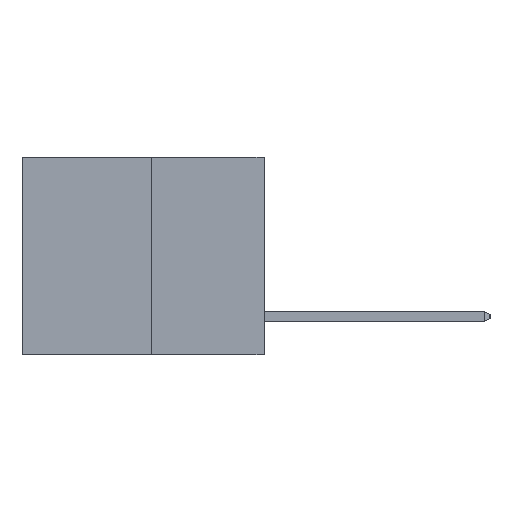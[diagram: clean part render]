
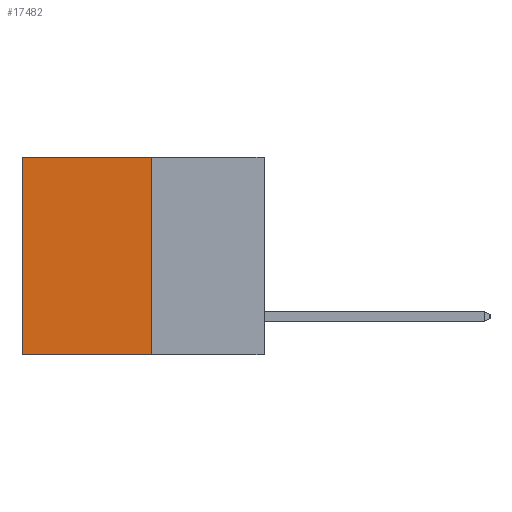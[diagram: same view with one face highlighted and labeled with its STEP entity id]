
A CAD part, left-side view. The second image highlights one B-rep face of the part: STEP entity #17482.
In plain terms, the highlighted planar face has unit normal (-1, 0, 0).
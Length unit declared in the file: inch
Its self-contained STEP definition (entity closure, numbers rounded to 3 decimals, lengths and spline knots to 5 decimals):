
#106 = ORIENTED_EDGE ( 'NONE', *, *, #21709, .F. ) ;
#440 = LINE ( 'NONE', #17711, #22484 ) ;
#1075 = CARTESIAN_POINT ( 'NONE',  ( 0.3165, 0.28, -0.49 ) ) ;
#2666 = DIRECTION ( 'NONE',  ( 0., 0., -1. ) ) ;
#2783 = EDGE_CURVE ( 'NONE', #6957, #25346, #440, .T. ) ;
#4240 = AXIS2_PLACEMENT_3D ( 'NONE', #26062, #8800, #26153 ) ;
#4554 = ORIENTED_EDGE ( 'NONE', *, *, #2783, .T. ) ;
#4633 = CARTESIAN_POINT ( 'NONE',  ( 0.3165, 0.28, 0. ) ) ;
#5804 = CARTESIAN_POINT ( 'NONE',  ( 0.3165, 0.28, 0. ) ) ;
#6434 = LINE ( 'NONE', #1075, #15392 ) ;
#6830 = EDGE_CURVE ( 'NONE', #8191, #25847, #21156, .T. ) ;
#6957 = VERTEX_POINT ( 'NONE', #19148 ) ;
#7073 = PLANE ( 'NONE',  #4240 ) ;
#8191 = VERTEX_POINT ( 'NONE', #5804 ) ;
#8423 = LINE ( 'NONE', #4633, #14415 ) ;
#8800 = DIRECTION ( 'NONE',  ( 1., 0., 0. ) ) ;
#9578 = CARTESIAN_POINT ( 'NONE',  ( 0.3165, 0.6, -0.49 ) ) ;
#11129 = ORIENTED_EDGE ( 'NONE', *, *, #6830, .F. ) ;
#13518 = EDGE_LOOP ( 'NONE', ( #4554, #106, #11129, #23353 ) ) ;
#14415 = VECTOR ( 'NONE', #17722, 39.37008 ) ;
#15269 = CARTESIAN_POINT ( 'NONE',  ( 0.3165, 0.28, -0.49 ) ) ;
#15392 = VECTOR ( 'NONE', #15847, 39.37008 ) ;
#15847 = DIRECTION ( 'NONE',  ( 0., 1., 0. ) ) ;
#15985 = CARTESIAN_POINT ( 'NONE',  ( 0.3165, 0.28, -0.49 ) ) ;
#17482 = ADVANCED_FACE ( 'NONE', ( #21801 ), #7073, .F. ) ;
#17711 = CARTESIAN_POINT ( 'NONE',  ( 0.3165, 0.6, -0.49 ) ) ;
#17722 = DIRECTION ( 'NONE',  ( 0., 1., 0. ) ) ;
#18143 = VECTOR ( 'NONE', #22916, 39.37008 ) ;
#19148 = CARTESIAN_POINT ( 'NONE',  ( 0.3165, 0.6, 0. ) ) ;
#21156 = LINE ( 'NONE', #15985, #18143 ) ;
#21499 = EDGE_CURVE ( 'NONE', #8191, #6957, #8423, .T. ) ;
#21709 = EDGE_CURVE ( 'NONE', #25847, #25346, #6434, .T. ) ;
#21801 = FACE_OUTER_BOUND ( 'NONE', #13518, .T. ) ;
#22484 = VECTOR ( 'NONE', #2666, 39.37008 ) ;
#22916 = DIRECTION ( 'NONE',  ( 0., 0., -1. ) ) ;
#23353 = ORIENTED_EDGE ( 'NONE', *, *, #21499, .T. ) ;
#25346 = VERTEX_POINT ( 'NONE', #9578 ) ;
#25847 = VERTEX_POINT ( 'NONE', #15269 ) ;
#26062 = CARTESIAN_POINT ( 'NONE',  ( 0.3165, 0.28, -0.49 ) ) ;
#26153 = DIRECTION ( 'NONE',  ( 0., 0., -1. ) ) ;
